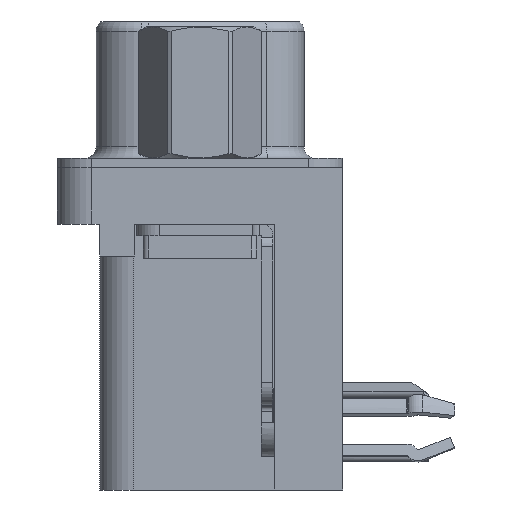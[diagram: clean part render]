
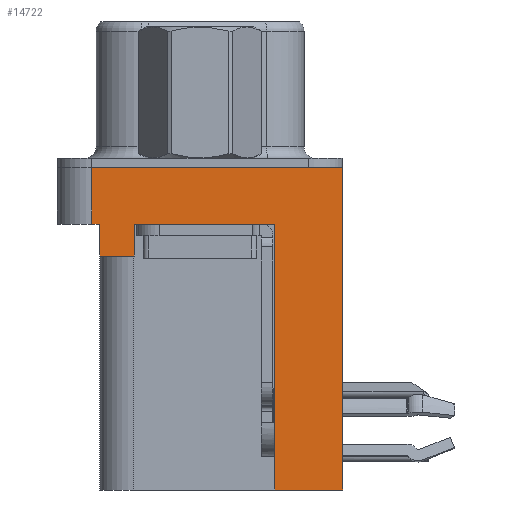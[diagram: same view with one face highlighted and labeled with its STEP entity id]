
A CAD part, left-side view. The second image highlights one B-rep face of the part: STEP entity #14722.
In plain terms, the highlighted planar face has unit normal (-1, 0, 0).
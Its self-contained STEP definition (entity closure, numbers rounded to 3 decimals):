
#150 = EDGE_CURVE ( 'NONE', #12405, #10935, #6540, .T. ) ;
#219 = DIRECTION ( 'NONE',  ( 0., -1., 0. ) ) ;
#703 = LINE ( 'NONE', #14804, #15653 ) ;
#1269 = ORIENTED_EDGE ( 'NONE', *, *, #13451, .T. ) ;
#1542 = EDGE_CURVE ( 'NONE', #17138, #16113, #16368, .T. ) ;
#1803 = VECTOR ( 'NONE', #21705, 1000. ) ;
#1869 = CARTESIAN_POINT ( 'NONE',  ( -2.91, -6.275, -2.5 ) ) ;
#1980 = LINE ( 'NONE', #1869, #5791 ) ;
#3139 = EDGE_CURVE ( 'NONE', #17138, #21108, #15069, .T. ) ;
#3629 = CARTESIAN_POINT ( 'NONE',  ( -2.91, -6.275, -14.2 ) ) ;
#3802 = CARTESIAN_POINT ( 'NONE',  ( -2.91, -6.275, 0. ) ) ;
#3905 = DIRECTION ( 'NONE',  ( 0., 1., 0. ) ) ;
#4443 = DIRECTION ( 'NONE',  ( 0., -1., 0. ) ) ;
#4752 = CARTESIAN_POINT ( 'NONE',  ( -2.91, -3.295, -14.2 ) ) ;
#4933 = VECTOR ( 'NONE', #18439, 1000. ) ;
#5170 = DIRECTION ( 'NONE',  ( 0., 1., 0. ) ) ;
#5212 = DIRECTION ( 'NONE',  ( 0., 0., 1. ) ) ;
#5490 = EDGE_CURVE ( 'NONE', #14313, #20983, #14419, .T. ) ;
#5791 = VECTOR ( 'NONE', #5212, 1000. ) ;
#6068 = VERTEX_POINT ( 'NONE', #9452 ) ;
#6300 = DIRECTION ( 'NONE',  ( 0., 0., 1. ) ) ;
#6540 = LINE ( 'NONE', #15216, #14952 ) ;
#7780 = LINE ( 'NONE', #14974, #4933 ) ;
#8003 = CARTESIAN_POINT ( 'NONE',  ( -2.91, -3.295, -2.5 ) ) ;
#8064 = VECTOR ( 'NONE', #4443, 1000. ) ;
#8092 = CARTESIAN_POINT ( 'NONE',  ( -2.91, -6.275, -2.5 ) ) ;
#8329 = ORIENTED_EDGE ( 'NONE', *, *, #17791, .F. ) ;
#8728 = EDGE_CURVE ( 'NONE', #20983, #15580, #17040, .T. ) ;
#9254 = ORIENTED_EDGE ( 'NONE', *, *, #1542, .F. ) ;
#9452 = CARTESIAN_POINT ( 'NONE',  ( -2.91, -6.275, 0. ) ) ;
#9567 = ORIENTED_EDGE ( 'NONE', *, *, #3139, .T. ) ;
#9898 = EDGE_LOOP ( 'NONE', ( #8329, #9254, #9567, #21199, #11472, #15742, #1269, #18881, #11850, #15474 ) ) ;
#10154 = DIRECTION ( 'NONE',  ( -1., 0., 0. ) ) ;
#10935 = VERTEX_POINT ( 'NONE', #16958 ) ;
#11429 = DIRECTION ( 'NONE',  ( 0., 0., 1. ) ) ;
#11472 = ORIENTED_EDGE ( 'NONE', *, *, #13151, .F. ) ;
#11850 = ORIENTED_EDGE ( 'NONE', *, *, #5490, .F. ) ;
#12201 = CARTESIAN_POINT ( 'NONE',  ( -2.91, 4.775, -2.5 ) ) ;
#12405 = VERTEX_POINT ( 'NONE', #12623 ) ;
#12453 = LINE ( 'NONE', #3802, #19178 ) ;
#12623 = CARTESIAN_POINT ( 'NONE',  ( -2.91, 2.895, -3.9 ) ) ;
#13050 = EDGE_CURVE ( 'NONE', #17952, #21108, #703, .T. ) ;
#13151 = EDGE_CURVE ( 'NONE', #12405, #17952, #14165, .T. ) ;
#13338 = CARTESIAN_POINT ( 'NONE',  ( -2.91, 4.425, -2.5 ) ) ;
#13424 = FACE_OUTER_BOUND ( 'NONE', #9898, .T. ) ;
#13451 = EDGE_CURVE ( 'NONE', #10935, #15580, #7780, .T. ) ;
#14165 = LINE ( 'NONE', #17625, #14932 ) ;
#14313 = VERTEX_POINT ( 'NONE', #3629 ) ;
#14419 = LINE ( 'NONE', #21484, #16319 ) ;
#14722 = ADVANCED_FACE ( 'NONE', ( #13424 ), #18871, .T. ) ;
#14804 = CARTESIAN_POINT ( 'NONE',  ( -2.91, 4.425, -3.9 ) ) ;
#14932 = VECTOR ( 'NONE', #5170, 1000. ) ;
#14939 = EDGE_CURVE ( 'NONE', #14313, #6068, #1980, .T. ) ;
#14952 = VECTOR ( 'NONE', #20321, 1000. ) ;
#14974 = CARTESIAN_POINT ( 'NONE',  ( -2.91, -6.275, -2.5 ) ) ;
#15069 = LINE ( 'NONE', #22138, #8064 ) ;
#15079 = CARTESIAN_POINT ( 'NONE',  ( -2.91, -3.295, -14.2 ) ) ;
#15173 = DIRECTION ( 'NONE',  ( 0., 0., 1. ) ) ;
#15216 = CARTESIAN_POINT ( 'NONE',  ( -2.91, 2.895, -3.9 ) ) ;
#15474 = ORIENTED_EDGE ( 'NONE', *, *, #14939, .T. ) ;
#15485 = CARTESIAN_POINT ( 'NONE',  ( -2.91, 4.775, 0. ) ) ;
#15580 = VERTEX_POINT ( 'NONE', #8003 ) ;
#15653 = VECTOR ( 'NONE', #11429, 1000. ) ;
#15742 = ORIENTED_EDGE ( 'NONE', *, *, #150, .T. ) ;
#15760 = AXIS2_PLACEMENT_3D ( 'NONE', #8092, #10154, #15173 ) ;
#16113 = VERTEX_POINT ( 'NONE', #15485 ) ;
#16265 = CARTESIAN_POINT ( 'NONE',  ( -2.91, 4.775, -2.5 ) ) ;
#16319 = VECTOR ( 'NONE', #3905, 1000. ) ;
#16368 = LINE ( 'NONE', #16265, #1803 ) ;
#16958 = CARTESIAN_POINT ( 'NONE',  ( -2.91, 2.895, -2.5 ) ) ;
#17040 = LINE ( 'NONE', #15079, #19195 ) ;
#17138 = VERTEX_POINT ( 'NONE', #12201 ) ;
#17625 = CARTESIAN_POINT ( 'NONE',  ( -2.91, 4.425, -3.9 ) ) ;
#17791 = EDGE_CURVE ( 'NONE', #16113, #6068, #12453, .T. ) ;
#17952 = VERTEX_POINT ( 'NONE', #18344 ) ;
#18344 = CARTESIAN_POINT ( 'NONE',  ( -2.91, 4.425, -3.9 ) ) ;
#18439 = DIRECTION ( 'NONE',  ( 0., -1., 0. ) ) ;
#18871 = PLANE ( 'NONE',  #15760 ) ;
#18881 = ORIENTED_EDGE ( 'NONE', *, *, #8728, .F. ) ;
#19178 = VECTOR ( 'NONE', #219, 1000. ) ;
#19195 = VECTOR ( 'NONE', #6300, 1000. ) ;
#20321 = DIRECTION ( 'NONE',  ( 0., 0., 1. ) ) ;
#20983 = VERTEX_POINT ( 'NONE', #4752 ) ;
#21108 = VERTEX_POINT ( 'NONE', #13338 ) ;
#21199 = ORIENTED_EDGE ( 'NONE', *, *, #13050, .F. ) ;
#21484 = CARTESIAN_POINT ( 'NONE',  ( -2.91, -3.295, -14.2 ) ) ;
#21705 = DIRECTION ( 'NONE',  ( 0., 0., 1. ) ) ;
#22138 = CARTESIAN_POINT ( 'NONE',  ( -2.91, -6.275, -2.5 ) ) ;
